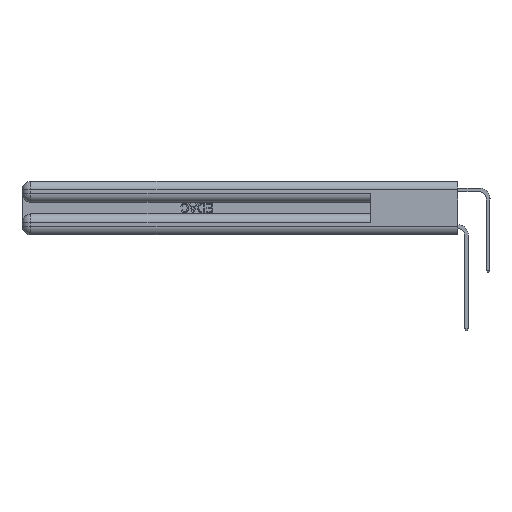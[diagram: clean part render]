
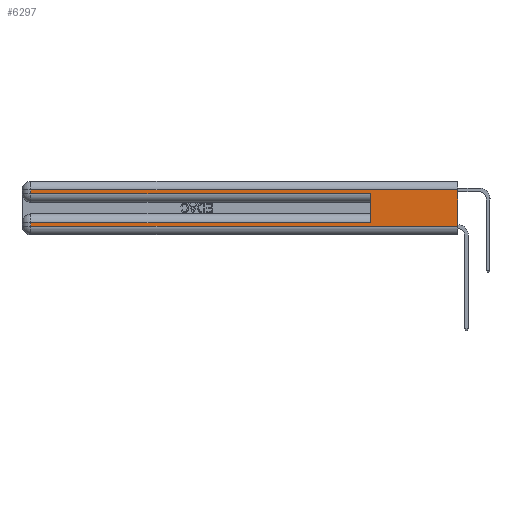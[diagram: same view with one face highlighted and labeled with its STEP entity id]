
A CAD part, left-side view. The second image highlights one B-rep face of the part: STEP entity #6297.
In plain terms, the highlighted planar face has unit normal (-1, 0, 0).
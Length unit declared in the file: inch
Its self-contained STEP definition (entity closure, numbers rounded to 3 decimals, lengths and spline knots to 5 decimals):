
#2751 = FACE_OUTER_BOUND ( 'NONE', #8061, .T. ) ;
#3408 = CARTESIAN_POINT ( 'NONE',  ( 0., 0., 0.31 ) ) ;
#3642 = LINE ( 'NONE', #11281, #33122 ) ;
#4046 = LINE ( 'NONE', #3408, #20028 ) ;
#5363 = DIRECTION ( 'NONE',  ( 0., 0., -1. ) ) ;
#6297 = ADVANCED_FACE ( 'NONE', ( #2751 ), #24826, .F. ) ;
#6933 = AXIS2_PLACEMENT_3D ( 'NONE', #30749, #13655, #33651 ) ;
#7159 = CARTESIAN_POINT ( 'NONE',  ( 0., 0., 0.37 ) ) ;
#7980 = LINE ( 'NONE', #30191, #32498 ) ;
#8061 = EDGE_LOOP ( 'NONE', ( #27231, #32404, #18064, #15815, #23270, #8536, #24739, #9754 ) ) ;
#8536 = ORIENTED_EDGE ( 'NONE', *, *, #34274, .T. ) ;
#9746 = EDGE_CURVE ( 'NONE', #33290, #29855, #14962, .T. ) ;
#9754 = ORIENTED_EDGE ( 'NONE', *, *, #31632, .T. ) ;
#10205 = VERTEX_POINT ( 'NONE', #17466 ) ;
#10505 = VERTEX_POINT ( 'NONE', #23903 ) ;
#11179 = DIRECTION ( 'NONE',  ( 0., 0., -1. ) ) ;
#11281 = CARTESIAN_POINT ( 'NONE',  ( 0., 0., 0.06 ) ) ;
#11584 = EDGE_CURVE ( 'NONE', #12398, #32186, #15535, .T. ) ;
#12150 = VECTOR ( 'NONE', #18531, 39.37008 ) ;
#12398 = VERTEX_POINT ( 'NONE', #21660 ) ;
#13590 = CARTESIAN_POINT ( 'NONE',  ( 0., 2.94, 0.285 ) ) ;
#13655 = DIRECTION ( 'NONE',  ( 1., 0., 0. ) ) ;
#14962 = LINE ( 'NONE', #36652, #29258 ) ;
#15535 = LINE ( 'NONE', #30908, #32989 ) ;
#15815 = ORIENTED_EDGE ( 'NONE', *, *, #19204, .T. ) ;
#15847 = CARTESIAN_POINT ( 'NONE',  ( 0., 0., 0.085 ) ) ;
#16320 = DIRECTION ( 'NONE',  ( 0., -1., 0. ) ) ;
#17466 = CARTESIAN_POINT ( 'NONE',  ( 0., 0.6, 0.085 ) ) ;
#17614 = LINE ( 'NONE', #25213, #18045 ) ;
#18045 = VECTOR ( 'NONE', #34871, 39.37008 ) ;
#18064 = ORIENTED_EDGE ( 'NONE', *, *, #11584, .T. ) ;
#18531 = DIRECTION ( 'NONE',  ( 0., 0., -1. ) ) ;
#19204 = EDGE_CURVE ( 'NONE', #32186, #25752, #17614, .T. ) ;
#19888 = VECTOR ( 'NONE', #21717, 39.37008 ) ;
#20028 = VECTOR ( 'NONE', #35360, 39.37008 ) ;
#21405 = EDGE_CURVE ( 'NONE', #10505, #25348, #34040, .T. ) ;
#21660 = CARTESIAN_POINT ( 'NONE',  ( 0., 2.94, 0.31 ) ) ;
#21717 = DIRECTION ( 'NONE',  ( 0., 1., 0. ) ) ;
#23269 = CARTESIAN_POINT ( 'NONE',  ( 0., 2.94, 0.06 ) ) ;
#23270 = ORIENTED_EDGE ( 'NONE', *, *, #23489, .F. ) ;
#23489 = EDGE_CURVE ( 'NONE', #10205, #25752, #7980, .T. ) ;
#23903 = CARTESIAN_POINT ( 'NONE',  ( 0., 0., 0.31 ) ) ;
#24167 = CARTESIAN_POINT ( 'NONE',  ( 0., 0., 0.06 ) ) ;
#24739 = ORIENTED_EDGE ( 'NONE', *, *, #9746, .T. ) ;
#24826 = PLANE ( 'NONE',  #6933 ) ;
#25213 = CARTESIAN_POINT ( 'NONE',  ( 0., 0., 0.285 ) ) ;
#25348 = VERTEX_POINT ( 'NONE', #24167 ) ;
#25752 = VERTEX_POINT ( 'NONE', #30228 ) ;
#27231 = ORIENTED_EDGE ( 'NONE', *, *, #21405, .F. ) ;
#29258 = VECTOR ( 'NONE', #11179, 39.37008 ) ;
#29767 = LINE ( 'NONE', #15847, #19888 ) ;
#29855 = VERTEX_POINT ( 'NONE', #23269 ) ;
#30191 = CARTESIAN_POINT ( 'NONE',  ( 0., 0.6, 0.145 ) ) ;
#30228 = CARTESIAN_POINT ( 'NONE',  ( 0., 0.6, 0.285 ) ) ;
#30749 = CARTESIAN_POINT ( 'NONE',  ( 0., 0., 0.37 ) ) ;
#30908 = CARTESIAN_POINT ( 'NONE',  ( 0., 2.94, 0.37 ) ) ;
#31632 = EDGE_CURVE ( 'NONE', #29855, #25348, #3642, .T. ) ;
#32186 = VERTEX_POINT ( 'NONE', #13590 ) ;
#32404 = ORIENTED_EDGE ( 'NONE', *, *, #32566, .T. ) ;
#32498 = VECTOR ( 'NONE', #33205, 39.37008 ) ;
#32566 = EDGE_CURVE ( 'NONE', #10505, #12398, #4046, .T. ) ;
#32989 = VECTOR ( 'NONE', #5363, 39.37008 ) ;
#33122 = VECTOR ( 'NONE', #16320, 39.37008 ) ;
#33205 = DIRECTION ( 'NONE',  ( 0., 0., 1. ) ) ;
#33290 = VERTEX_POINT ( 'NONE', #34945 ) ;
#33651 = DIRECTION ( 'NONE',  ( 0., 0., -1. ) ) ;
#34040 = LINE ( 'NONE', #7159, #12150 ) ;
#34274 = EDGE_CURVE ( 'NONE', #10205, #33290, #29767, .T. ) ;
#34871 = DIRECTION ( 'NONE',  ( 0., -1., 0. ) ) ;
#34945 = CARTESIAN_POINT ( 'NONE',  ( 0., 2.94, 0.085 ) ) ;
#35360 = DIRECTION ( 'NONE',  ( 0., 1., 0. ) ) ;
#36652 = CARTESIAN_POINT ( 'NONE',  ( 0., 2.94, 0.37 ) ) ;
